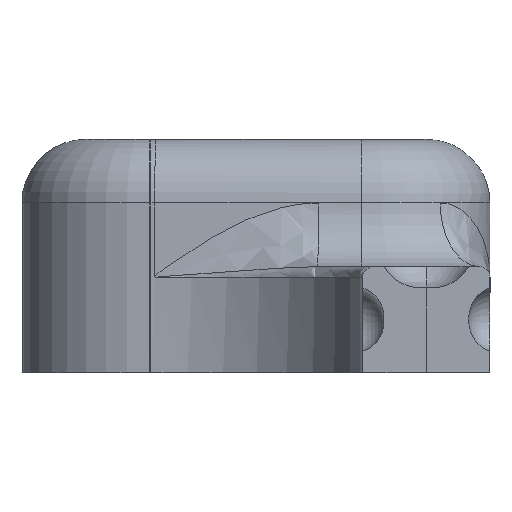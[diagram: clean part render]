
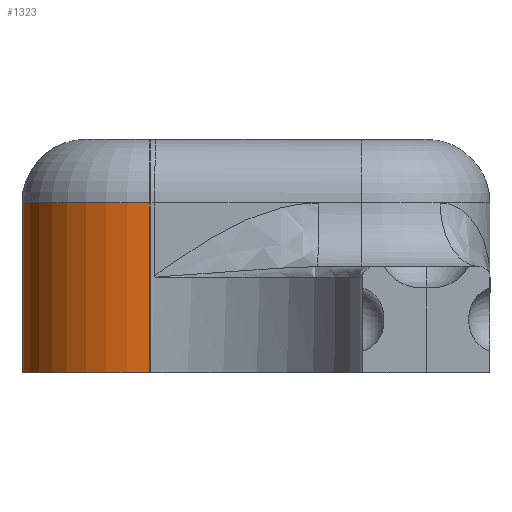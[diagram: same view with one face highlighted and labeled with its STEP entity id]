
A CAD part, left-side view. The second image highlights one B-rep face of the part: STEP entity #1323.
In plain terms, the highlighted cylindrical face has radius 6 mm (diameter 12 mm), a partial arc.
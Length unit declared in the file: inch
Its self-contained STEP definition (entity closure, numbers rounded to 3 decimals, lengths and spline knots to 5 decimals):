
#24 = CARTESIAN_POINT ( 'NONE',  ( 6.55004, 0.04269, -2.6378 ) ) ;
#79 = CARTESIAN_POINT ( 'NONE',  ( 6.55004, 0.04269, -2.75591 ) ) ;
#150 = CARTESIAN_POINT ( 'NONE',  ( 6.31381, 0.04269, -2.95276 ) ) ;
#220 = VECTOR ( 'NONE', #673, 39.37008 ) ;
#300 = DIRECTION ( 'NONE',  ( 1., 0., 0. ) ) ;
#347 = CARTESIAN_POINT ( 'NONE',  ( 6.55004, 0.04269, -2.95276 ) ) ;
#359 = FACE_OUTER_BOUND ( 'NONE', #887, .T. ) ;
#384 = CARTESIAN_POINT ( 'NONE',  ( 6.07759, 0.04269, -2.75591 ) ) ;
#407 = EDGE_CURVE ( 'NONE', #1278, #1354, #614, .T. ) ;
#432 = CARTESIAN_POINT ( 'NONE',  ( 6.07759, 0.04269, -2.6378 ) ) ;
#452 = EDGE_CURVE ( 'NONE', #937, #1450, #1274, .T. ) ;
#475 = DIRECTION ( 'NONE',  ( 1., 0., 0. ) ) ;
#506 = AXIS2_PLACEMENT_3D ( 'NONE', #613, #1583, #764 ) ;
#518 = EDGE_CURVE ( 'NONE', #1354, #1450, #1512, .T. ) ;
#573 = AXIS2_PLACEMENT_3D ( 'NONE', #638, #789, #475 ) ;
#613 = CARTESIAN_POINT ( 'NONE',  ( 6.31381, 0.04269, -2.6378 ) ) ;
#614 = LINE ( 'NONE', #79, #220 ) ;
#638 = CARTESIAN_POINT ( 'NONE',  ( 6.31381, 0.04269, -2.75591 ) ) ;
#673 = DIRECTION ( 'NONE',  ( 0., 0., -1. ) ) ;
#688 = AXIS2_PLACEMENT_3D ( 'NONE', #150, #1164, #300 ) ;
#764 = DIRECTION ( 'NONE',  ( -1., 0., 0. ) ) ;
#789 = DIRECTION ( 'NONE',  ( 0., 0., -1. ) ) ;
#887 = EDGE_LOOP ( 'NONE', ( #1516, #996, #1271, #1405 ) ) ;
#937 = VERTEX_POINT ( 'NONE', #432 ) ;
#996 = ORIENTED_EDGE ( 'NONE', *, *, #1190, .T. ) ;
#1164 = DIRECTION ( 'NONE',  ( 0., 0., 1. ) ) ;
#1190 = EDGE_CURVE ( 'NONE', #937, #1278, #1264, .T. ) ;
#1233 = VECTOR ( 'NONE', #1241, 39.37008 ) ;
#1241 = DIRECTION ( 'NONE',  ( 0., 0., -1. ) ) ;
#1264 = CIRCLE ( 'NONE', #506, 0.23622 ) ;
#1271 = ORIENTED_EDGE ( 'NONE', *, *, #407, .T. ) ;
#1274 = LINE ( 'NONE', #384, #1233 ) ;
#1278 = VERTEX_POINT ( 'NONE', #24 ) ;
#1323 = ADVANCED_FACE ( 'NONE', ( #359 ), #1411, .T. ) ;
#1354 = VERTEX_POINT ( 'NONE', #347 ) ;
#1405 = ORIENTED_EDGE ( 'NONE', *, *, #518, .T. ) ;
#1411 = CYLINDRICAL_SURFACE ( 'NONE', #573, 0.23622 ) ;
#1450 = VERTEX_POINT ( 'NONE', #1486 ) ;
#1486 = CARTESIAN_POINT ( 'NONE',  ( 6.07759, 0.04269, -2.95276 ) ) ;
#1512 = CIRCLE ( 'NONE', #688, 0.23622 ) ;
#1516 = ORIENTED_EDGE ( 'NONE', *, *, #452, .F. ) ;
#1583 = DIRECTION ( 'NONE',  ( 0., 0., -1. ) ) ;
